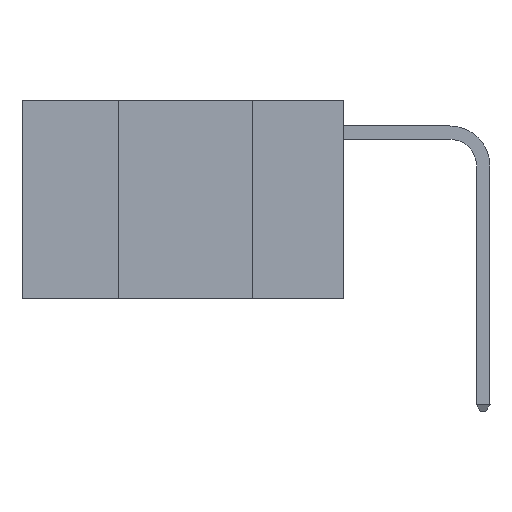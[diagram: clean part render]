
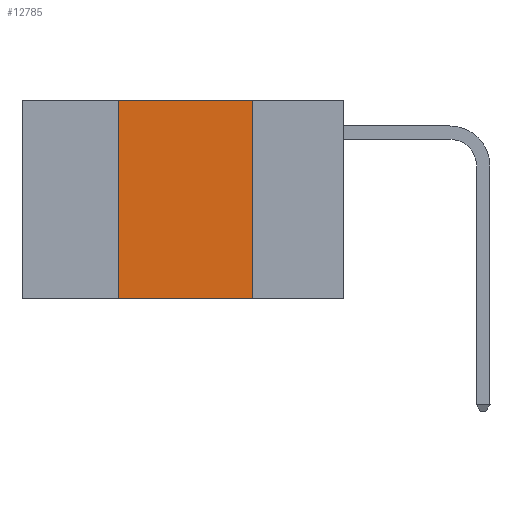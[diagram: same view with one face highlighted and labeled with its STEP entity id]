
A CAD part, left-side view. The second image highlights one B-rep face of the part: STEP entity #12785.
In plain terms, the highlighted planar face has unit normal (-1, 0, 0).
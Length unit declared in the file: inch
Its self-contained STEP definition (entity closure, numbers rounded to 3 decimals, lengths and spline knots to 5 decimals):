
#356 = ORIENTED_EDGE ( 'NONE', *, *, #1748, .F. ) ;
#419 = ORIENTED_EDGE ( 'NONE', *, *, #7558, .F. ) ;
#449 = ORIENTED_EDGE ( 'NONE', *, *, #2066, .F. ) ;
#534 = ORIENTED_EDGE ( 'NONE', *, *, #1608, .T. ) ;
#1230 = AXIS2_PLACEMENT_3D ( 'NONE', #13439, #6425, #14525 ) ;
#1406 = CARTESIAN_POINT ( 'NONE',  ( 0., 0.42, 0. ) ) ;
#1608 = EDGE_CURVE ( 'NONE', #7504, #3593, #2761, .T. ) ;
#1748 = EDGE_CURVE ( 'NONE', #6057, #3593, #1842, .T. ) ;
#1770 = VECTOR ( 'NONE', #7410, 39.37008 ) ;
#1842 = LINE ( 'NONE', #7535, #1770 ) ;
#2066 = EDGE_CURVE ( 'NONE', #7504, #9074, #14201, .T. ) ;
#2092 = LINE ( 'NONE', #9552, #13286 ) ;
#2761 = LINE ( 'NONE', #8689, #2870 ) ;
#2870 = VECTOR ( 'NONE', #8671, 39.37008 ) ;
#3231 = CARTESIAN_POINT ( 'NONE',  ( 0., 0.17, -0.37 ) ) ;
#3593 = VERTEX_POINT ( 'NONE', #3231 ) ;
#4642 = CARTESIAN_POINT ( 'NONE',  ( 0., 0.42, -0.37 ) ) ;
#4755 = DIRECTION ( 'NONE',  ( 0., -1., 0. ) ) ;
#4956 = DIRECTION ( 'NONE',  ( 0., 0., 1. ) ) ;
#5071 = CARTESIAN_POINT ( 'NONE',  ( 0., 0.42, 0. ) ) ;
#6057 = VERTEX_POINT ( 'NONE', #9438 ) ;
#6425 = DIRECTION ( 'NONE',  ( 1., 0., 0. ) ) ;
#7401 = FACE_OUTER_BOUND ( 'NONE', #9191, .T. ) ;
#7410 = DIRECTION ( 'NONE',  ( 0., 0., -1. ) ) ;
#7504 = VERTEX_POINT ( 'NONE', #4642 ) ;
#7535 = CARTESIAN_POINT ( 'NONE',  ( 0., 0.17, 0. ) ) ;
#7558 = EDGE_CURVE ( 'NONE', #9074, #6057, #2092, .T. ) ;
#8671 = DIRECTION ( 'NONE',  ( 0., -1., 0. ) ) ;
#8689 = CARTESIAN_POINT ( 'NONE',  ( 0., 0.6, -0.37 ) ) ;
#9074 = VERTEX_POINT ( 'NONE', #1406 ) ;
#9191 = EDGE_LOOP ( 'NONE', ( #356, #419, #449, #534 ) ) ;
#9438 = CARTESIAN_POINT ( 'NONE',  ( 0., 0.17, 0. ) ) ;
#9552 = CARTESIAN_POINT ( 'NONE',  ( 0., 0.6, 0. ) ) ;
#9975 = PLANE ( 'NONE',  #1230 ) ;
#12785 = ADVANCED_FACE ( 'NONE', ( #7401 ), #9975, .F. ) ;
#13286 = VECTOR ( 'NONE', #4755, 39.37008 ) ;
#13439 = CARTESIAN_POINT ( 'NONE',  ( 0., 0.6, 0. ) ) ;
#14103 = VECTOR ( 'NONE', #4956, 39.37008 ) ;
#14201 = LINE ( 'NONE', #5071, #14103 ) ;
#14525 = DIRECTION ( 'NONE',  ( 0., 0., -1. ) ) ;
